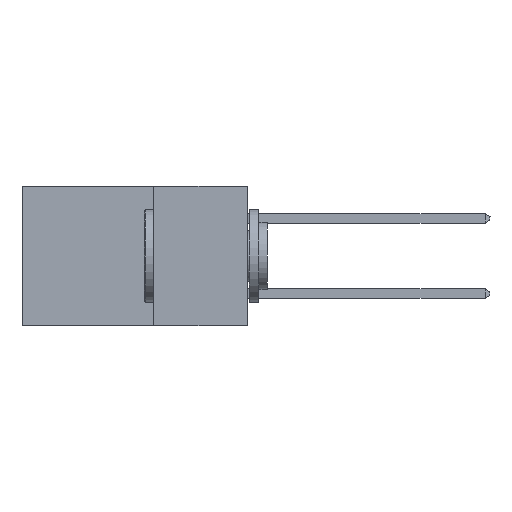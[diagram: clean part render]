
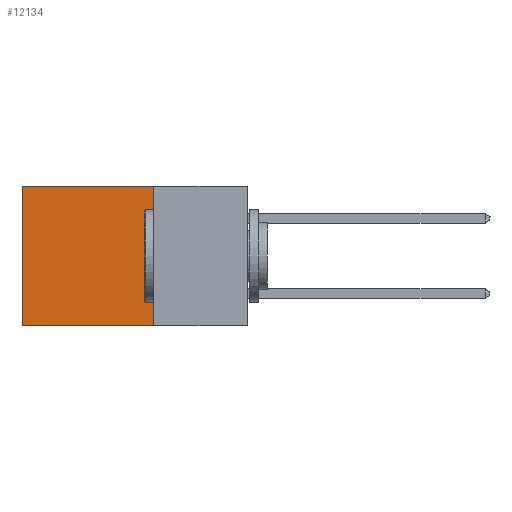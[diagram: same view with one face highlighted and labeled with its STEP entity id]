
A CAD part, left-side view. The second image highlights one B-rep face of the part: STEP entity #12134.
In plain terms, the highlighted planar face has unit normal (-1, 0, 0).
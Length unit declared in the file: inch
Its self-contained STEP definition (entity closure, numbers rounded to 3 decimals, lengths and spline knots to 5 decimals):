
#836 = VERTEX_POINT ( 'NONE', #11423 ) ;
#2026 = CARTESIAN_POINT ( 'NONE',  ( 0.298, 0.6, 0. ) ) ;
#2960 = ORIENTED_EDGE ( 'NONE', *, *, #8975, .F. ) ;
#3875 = EDGE_CURVE ( 'NONE', #21957, #836, #8218, .T. ) ;
#5423 = PLANE ( 'NONE',  #13151 ) ;
#8048 = DIRECTION ( 'NONE',  ( 0., 0., -1. ) ) ;
#8073 = FACE_OUTER_BOUND ( 'NONE', #26048, .T. ) ;
#8218 = LINE ( 'NONE', #22608, #13578 ) ;
#8246 = LINE ( 'NONE', #28404, #29894 ) ;
#8975 = EDGE_CURVE ( 'NONE', #25186, #21957, #22604, .T. ) ;
#9105 = VECTOR ( 'NONE', #22499, 39.37008 ) ;
#9536 = EDGE_CURVE ( 'NONE', #25186, #9840, #14423, .T. ) ;
#9840 = VERTEX_POINT ( 'NONE', #2026 ) ;
#10924 = DIRECTION ( 'NONE',  ( 0., 1., 0. ) ) ;
#11423 = CARTESIAN_POINT ( 'NONE',  ( 0.298, 0.6, -0.37 ) ) ;
#12134 = ADVANCED_FACE ( 'NONE', ( #8073 ), #5423, .F. ) ;
#13151 = AXIS2_PLACEMENT_3D ( 'NONE', #23725, #13589, #8048 ) ;
#13578 = VECTOR ( 'NONE', #14988, 39.37008 ) ;
#13589 = DIRECTION ( 'NONE',  ( 1., 0., 0. ) ) ;
#14423 = LINE ( 'NONE', #26554, #29889 ) ;
#14988 = DIRECTION ( 'NONE',  ( 0., 1., 0. ) ) ;
#16184 = ORIENTED_EDGE ( 'NONE', *, *, #31363, .T. ) ;
#19989 = CARTESIAN_POINT ( 'NONE',  ( 0.298, 0.25, 0. ) ) ;
#21549 = ORIENTED_EDGE ( 'NONE', *, *, #9536, .T. ) ;
#21957 = VERTEX_POINT ( 'NONE', #24609 ) ;
#22499 = DIRECTION ( 'NONE',  ( 0., 0., -1. ) ) ;
#22604 = LINE ( 'NONE', #19989, #9105 ) ;
#22608 = CARTESIAN_POINT ( 'NONE',  ( 0.298, 0.25, -0.37 ) ) ;
#23725 = CARTESIAN_POINT ( 'NONE',  ( 0.298, 0.25, 0. ) ) ;
#24082 = ORIENTED_EDGE ( 'NONE', *, *, #3875, .F. ) ;
#24609 = CARTESIAN_POINT ( 'NONE',  ( 0.298, 0.25, -0.37 ) ) ;
#25186 = VERTEX_POINT ( 'NONE', #25261 ) ;
#25261 = CARTESIAN_POINT ( 'NONE',  ( 0.298, 0.25, 0. ) ) ;
#26048 = EDGE_LOOP ( 'NONE', ( #16184, #24082, #2960, #21549 ) ) ;
#26554 = CARTESIAN_POINT ( 'NONE',  ( 0.298, 0.25, 0. ) ) ;
#28404 = CARTESIAN_POINT ( 'NONE',  ( 0.298, 0.6, 0. ) ) ;
#29889 = VECTOR ( 'NONE', #10924, 39.37008 ) ;
#29894 = VECTOR ( 'NONE', #33702, 39.37008 ) ;
#31363 = EDGE_CURVE ( 'NONE', #9840, #836, #8246, .T. ) ;
#33702 = DIRECTION ( 'NONE',  ( 0., 0., -1. ) ) ;
